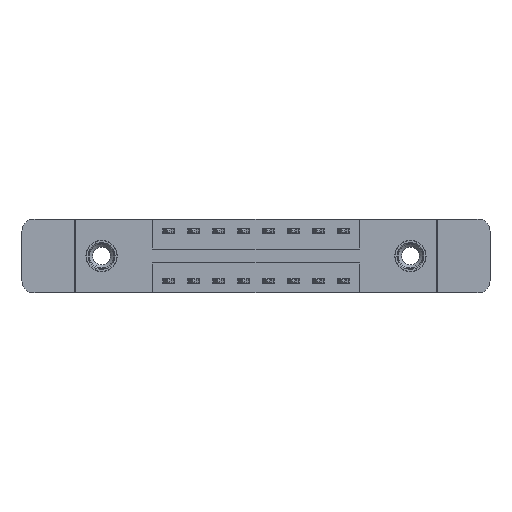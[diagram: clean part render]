
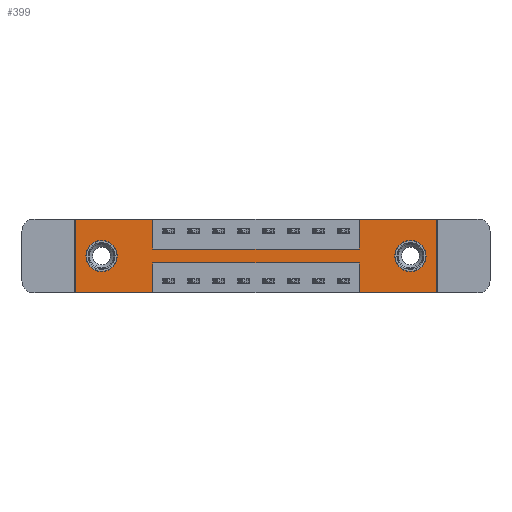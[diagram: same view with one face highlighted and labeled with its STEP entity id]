
A CAD part, front view. The second image highlights one B-rep face of the part: STEP entity #399.
In plain terms, the highlighted planar face has unit normal (0, -1, 0).
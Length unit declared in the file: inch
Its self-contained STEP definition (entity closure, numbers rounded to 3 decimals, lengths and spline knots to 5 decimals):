
#100 = CARTESIAN_POINT ( 'NONE',  ( 1.81, 0., 0. ) ) ;
#138 = VECTOR ( 'NONE', #3414, 39.37008 ) ;
#385 = DIRECTION ( 'NONE',  ( 0., -1., 0. ) ) ;
#399 = ADVANCED_FACE ( 'NONE', ( #9846, #9674, #5892 ), #14273, .T. ) ;
#566 = VERTEX_POINT ( 'NONE', #3155 ) ;
#579 = DIRECTION ( 'NONE',  ( 0., 0., 1. ) ) ;
#613 = CARTESIAN_POINT ( 'NONE',  ( 0., 0., 0. ) ) ;
#653 = ORIENTED_EDGE ( 'NONE', *, *, #11011, .T. ) ;
#707 = VECTOR ( 'NONE', #14963, 39.37008 ) ;
#760 = DIRECTION ( 'NONE',  ( 1., 0., 0. ) ) ;
#795 = DIRECTION ( 'NONE',  ( 0., 0., -1. ) ) ;
#938 = EDGE_CURVE ( 'NONE', #7951, #566, #2452, .T. ) ;
#1016 = DIRECTION ( 'NONE',  ( 0., 0., -1. ) ) ;
#1730 = LINE ( 'NONE', #6824, #138 ) ;
#1789 = EDGE_CURVE ( 'NONE', #12554, #11698, #2793, .T. ) ;
#1854 = CARTESIAN_POINT ( 'NONE',  ( 0., 0., 0. ) ) ;
#1861 = DIRECTION ( 'NONE',  ( 0., 0., -1. ) ) ;
#1913 = VERTEX_POINT ( 'NONE', #10922 ) ;
#1973 = CARTESIAN_POINT ( 'NONE',  ( 0., 0., -0.37 ) ) ;
#2074 = DIRECTION ( 'NONE',  ( 0., 1., 0. ) ) ;
#2313 = ORIENTED_EDGE ( 'NONE', *, *, #14566, .F. ) ;
#2337 = ORIENTED_EDGE ( 'NONE', *, *, #8176, .F. ) ;
#2452 = CIRCLE ( 'NONE', #10619, 0.078 ) ;
#2588 = AXIS2_PLACEMENT_3D ( 'NONE', #11032, #6350, #579 ) ;
#2697 = AXIS2_PLACEMENT_3D ( 'NONE', #13118, #385, #9680 ) ;
#2793 = LINE ( 'NONE', #100, #14758 ) ;
#2910 = AXIS2_PLACEMENT_3D ( 'NONE', #3305, #5627, #10147 ) ;
#2931 = ORIENTED_EDGE ( 'NONE', *, *, #10503, .F. ) ;
#3155 = CARTESIAN_POINT ( 'NONE',  ( 1.6775, 0., -0.263 ) ) ;
#3305 = CARTESIAN_POINT ( 'NONE',  ( 1.6775, 0., -0.185 ) ) ;
#3402 = ORIENTED_EDGE ( 'NONE', *, *, #11183, .F. ) ;
#3414 = DIRECTION ( 'NONE',  ( -1., 0., 0. ) ) ;
#3510 = CIRCLE ( 'NONE', #2910, 0.078 ) ;
#3619 = CARTESIAN_POINT ( 'NONE',  ( 0.3875, 0., -0.37 ) ) ;
#3808 = CARTESIAN_POINT ( 'NONE',  ( 1.6775, 0., -0.107 ) ) ;
#3843 = CARTESIAN_POINT ( 'NONE',  ( 0.1325, 0., -0.107 ) ) ;
#3888 = VECTOR ( 'NONE', #6527, 39.37008 ) ;
#3934 = DIRECTION ( 'NONE',  ( -1., 0., 0. ) ) ;
#4168 = LINE ( 'NONE', #8492, #707 ) ;
#4185 = EDGE_CURVE ( 'NONE', #12883, #10958, #10628, .T. ) ;
#4201 = CARTESIAN_POINT ( 'NONE',  ( 0.1325, 0., -0.185 ) ) ;
#5342 = CARTESIAN_POINT ( 'NONE',  ( 1.4225, 0., -0.37 ) ) ;
#5386 = CARTESIAN_POINT ( 'NONE',  ( 0., 0., -0.37 ) ) ;
#5530 = DIRECTION ( 'NONE',  ( 0., 1., 0. ) ) ;
#5605 = CARTESIAN_POINT ( 'NONE',  ( 0.3875, 0., -0.15 ) ) ;
#5627 = DIRECTION ( 'NONE',  ( 0., 1., 0. ) ) ;
#5677 = VERTEX_POINT ( 'NONE', #3619 ) ;
#5705 = CARTESIAN_POINT ( 'NONE',  ( 1.4225, 0., -0.37 ) ) ;
#5892 = FACE_OUTER_BOUND ( 'NONE', #14283, .T. ) ;
#5903 = EDGE_LOOP ( 'NONE', ( #6715, #653 ) ) ;
#6161 = EDGE_CURVE ( 'NONE', #6572, #14430, #11297, .T. ) ;
#6350 = DIRECTION ( 'NONE',  ( 0., 1., 0. ) ) ;
#6393 = CARTESIAN_POINT ( 'NONE',  ( 0.3875, 0., 0. ) ) ;
#6527 = DIRECTION ( 'NONE',  ( -1., 0., 0. ) ) ;
#6572 = VERTEX_POINT ( 'NONE', #8514 ) ;
#6687 = DIRECTION ( 'NONE',  ( 1., 0., 0. ) ) ;
#6715 = ORIENTED_EDGE ( 'NONE', *, *, #938, .T. ) ;
#6824 = CARTESIAN_POINT ( 'NONE',  ( 0., 0., -0.37 ) ) ;
#6833 = EDGE_CURVE ( 'NONE', #5677, #12883, #7447, .T. ) ;
#6904 = ORIENTED_EDGE ( 'NONE', *, *, #8969, .F. ) ;
#7043 = ORIENTED_EDGE ( 'NONE', *, *, #8416, .T. ) ;
#7181 = CARTESIAN_POINT ( 'NONE',  ( 1.4225, 0., 0. ) ) ;
#7329 = DIRECTION ( 'NONE',  ( 0., 0., 1. ) ) ;
#7447 = LINE ( 'NONE', #5386, #3888 ) ;
#7860 = CARTESIAN_POINT ( 'NONE',  ( 0.3875, 0., -0.37 ) ) ;
#7951 = VERTEX_POINT ( 'NONE', #3808 ) ;
#8032 = VECTOR ( 'NONE', #7329, 39.37008 ) ;
#8119 = CARTESIAN_POINT ( 'NONE',  ( 0.3875, 0., -0.22 ) ) ;
#8143 = VECTOR ( 'NONE', #6687, 39.37008 ) ;
#8176 = EDGE_CURVE ( 'NONE', #9801, #5677, #11055, .T. ) ;
#8220 = DIRECTION ( 'NONE',  ( 0., 0., 1. ) ) ;
#8416 = EDGE_CURVE ( 'NONE', #14430, #6572, #9276, .T. ) ;
#8492 = CARTESIAN_POINT ( 'NONE',  ( 0., 0., 0. ) ) ;
#8514 = CARTESIAN_POINT ( 'NONE',  ( 0.1325, 0., -0.263 ) ) ;
#8613 = EDGE_CURVE ( 'NONE', #8795, #9761, #10671, .T. ) ;
#8765 = VERTEX_POINT ( 'NONE', #5605 ) ;
#8795 = VERTEX_POINT ( 'NONE', #5342 ) ;
#8842 = VECTOR ( 'NONE', #3934, 39.37008 ) ;
#8857 = CARTESIAN_POINT ( 'NONE',  ( 1.6775, 0., -0.185 ) ) ;
#8911 = ORIENTED_EDGE ( 'NONE', *, *, #10397, .F. ) ;
#8950 = EDGE_LOOP ( 'NONE', ( #7043, #11813 ) ) ;
#8969 = EDGE_CURVE ( 'NONE', #8765, #12432, #12291, .T. ) ;
#9005 = CARTESIAN_POINT ( 'NONE',  ( 1.81, 0., -0.37 ) ) ;
#9073 = CARTESIAN_POINT ( 'NONE',  ( 1.81, 0., 0. ) ) ;
#9152 = CARTESIAN_POINT ( 'NONE',  ( 0., 0., 0. ) ) ;
#9276 = CIRCLE ( 'NONE', #2588, 0.078 ) ;
#9602 = LINE ( 'NONE', #6393, #13042 ) ;
#9674 = FACE_BOUND ( 'NONE', #8950, .T. ) ;
#9680 = DIRECTION ( 'NONE',  ( 0., 0., -1. ) ) ;
#9761 = VERTEX_POINT ( 'NONE', #12675 ) ;
#9801 = VERTEX_POINT ( 'NONE', #8119 ) ;
#9846 = FACE_BOUND ( 'NONE', #5903, .T. ) ;
#10010 = EDGE_CURVE ( 'NONE', #1913, #12554, #11200, .T. ) ;
#10147 = DIRECTION ( 'NONE',  ( 0., 0., -1. ) ) ;
#10397 = EDGE_CURVE ( 'NONE', #10958, #14965, #4168, .T. ) ;
#10437 = ORIENTED_EDGE ( 'NONE', *, *, #13774, .F. ) ;
#10503 = EDGE_CURVE ( 'NONE', #12432, #1913, #12575, .T. ) ;
#10619 = AXIS2_PLACEMENT_3D ( 'NONE', #8857, #2074, #1861 ) ;
#10628 = LINE ( 'NONE', #613, #11164 ) ;
#10671 = LINE ( 'NONE', #5705, #14897 ) ;
#10730 = ORIENTED_EDGE ( 'NONE', *, *, #10010, .F. ) ;
#10922 = CARTESIAN_POINT ( 'NONE',  ( 1.4225, 0., 0. ) ) ;
#10958 = VERTEX_POINT ( 'NONE', #1854 ) ;
#11011 = EDGE_CURVE ( 'NONE', #566, #7951, #3510, .T. ) ;
#11032 = CARTESIAN_POINT ( 'NONE',  ( 0.1325, 0., -0.185 ) ) ;
#11055 = LINE ( 'NONE', #7860, #12527 ) ;
#11164 = VECTOR ( 'NONE', #8220, 39.37008 ) ;
#11183 = EDGE_CURVE ( 'NONE', #14965, #8765, #9602, .T. ) ;
#11200 = LINE ( 'NONE', #9152, #8143 ) ;
#11202 = CARTESIAN_POINT ( 'NONE',  ( 0.3875, 0., -0.15 ) ) ;
#11297 = CIRCLE ( 'NONE', #13711, 0.078 ) ;
#11638 = ORIENTED_EDGE ( 'NONE', *, *, #1789, .F. ) ;
#11698 = VERTEX_POINT ( 'NONE', #9005 ) ;
#11813 = ORIENTED_EDGE ( 'NONE', *, *, #6161, .T. ) ;
#11936 = ORIENTED_EDGE ( 'NONE', *, *, #6833, .F. ) ;
#12084 = CARTESIAN_POINT ( 'NONE',  ( 0.3875, 0., 0. ) ) ;
#12291 = LINE ( 'NONE', #11202, #13408 ) ;
#12432 = VERTEX_POINT ( 'NONE', #13249 ) ;
#12527 = VECTOR ( 'NONE', #1016, 39.37008 ) ;
#12554 = VERTEX_POINT ( 'NONE', #9073 ) ;
#12575 = LINE ( 'NONE', #7181, #8032 ) ;
#12675 = CARTESIAN_POINT ( 'NONE',  ( 1.4225, 0., -0.22 ) ) ;
#12883 = VERTEX_POINT ( 'NONE', #1973 ) ;
#13027 = ORIENTED_EDGE ( 'NONE', *, *, #4185, .F. ) ;
#13042 = VECTOR ( 'NONE', #14514, 39.37008 ) ;
#13118 = CARTESIAN_POINT ( 'NONE',  ( 0., 0., -0.37 ) ) ;
#13249 = CARTESIAN_POINT ( 'NONE',  ( 1.4225, 0., -0.15 ) ) ;
#13408 = VECTOR ( 'NONE', #760, 39.37008 ) ;
#13711 = AXIS2_PLACEMENT_3D ( 'NONE', #4201, #5530, #14583 ) ;
#13759 = CARTESIAN_POINT ( 'NONE',  ( 0.3875, 0., -0.22 ) ) ;
#13774 = EDGE_CURVE ( 'NONE', #9761, #9801, #14662, .T. ) ;
#13960 = DIRECTION ( 'NONE',  ( 0., 0., 1. ) ) ;
#14273 = PLANE ( 'NONE',  #2697 ) ;
#14283 = EDGE_LOOP ( 'NONE', ( #2337, #10437, #14693, #2313, #11638, #10730, #2931, #6904, #3402, #8911, #13027, #11936 ) ) ;
#14430 = VERTEX_POINT ( 'NONE', #3843 ) ;
#14514 = DIRECTION ( 'NONE',  ( 0., 0., -1. ) ) ;
#14566 = EDGE_CURVE ( 'NONE', #11698, #8795, #1730, .T. ) ;
#14583 = DIRECTION ( 'NONE',  ( 0., 0., 1. ) ) ;
#14662 = LINE ( 'NONE', #13759, #8842 ) ;
#14693 = ORIENTED_EDGE ( 'NONE', *, *, #8613, .F. ) ;
#14758 = VECTOR ( 'NONE', #795, 39.37008 ) ;
#14897 = VECTOR ( 'NONE', #13960, 39.37008 ) ;
#14963 = DIRECTION ( 'NONE',  ( 1., 0., 0. ) ) ;
#14965 = VERTEX_POINT ( 'NONE', #12084 ) ;
